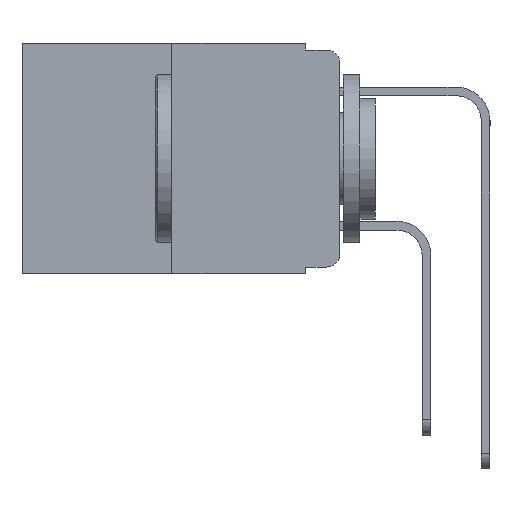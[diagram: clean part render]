
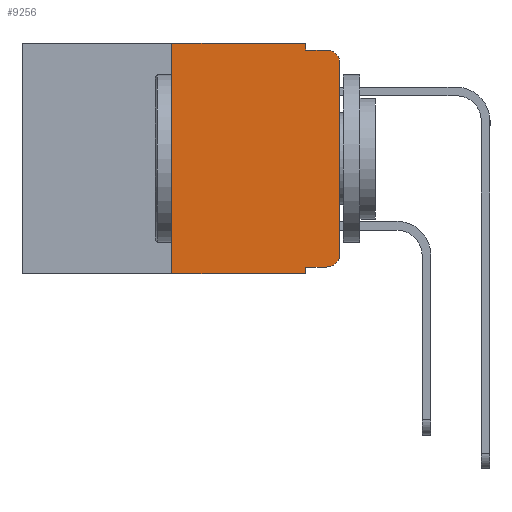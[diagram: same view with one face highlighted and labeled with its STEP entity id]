
A CAD part, left-side view. The second image highlights one B-rep face of the part: STEP entity #9256.
In plain terms, the highlighted planar face has unit normal (-1, 0, 0).
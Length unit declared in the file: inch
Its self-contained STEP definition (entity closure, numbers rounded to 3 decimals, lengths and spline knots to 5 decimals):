
#38 = LINE ( 'NONE', #16560, #7123 ) ;
#275 = CARTESIAN_POINT ( 'NONE',  ( 0., 0., 0. ) ) ;
#392 = LINE ( 'NONE', #10091, #4179 ) ;
#503 = EDGE_CURVE ( 'NONE', #14388, #8010, #17808, .T. ) ;
#567 = DIRECTION ( 'NONE',  ( 0., 0., -1. ) ) ;
#892 = EDGE_CURVE ( 'NONE', #16845, #3179, #9210, .T. ) ;
#1469 = CARTESIAN_POINT ( 'NONE',  ( 0., 0.473, 0. ) ) ;
#1489 = EDGE_CURVE ( 'NONE', #12962, #1530, #3821, .T. ) ;
#1524 = EDGE_CURVE ( 'NONE', #1530, #16485, #10267, .T. ) ;
#1530 = VERTEX_POINT ( 'NONE', #8694 ) ;
#1806 = DIRECTION ( 'NONE',  ( 0., 0., 1. ) ) ;
#2281 = ORIENTED_EDGE ( 'NONE', *, *, #11117, .T. ) ;
#2310 = VECTOR ( 'NONE', #11125, 39.37008 ) ;
#2335 = DIRECTION ( 'NONE',  ( 0., -1., 0. ) ) ;
#2382 = VERTEX_POINT ( 'NONE', #11726 ) ;
#2579 = EDGE_CURVE ( 'NONE', #4238, #16485, #3986, .T. ) ;
#2653 = DIRECTION ( 'NONE',  ( 0., 0., -1. ) ) ;
#3179 = VERTEX_POINT ( 'NONE', #8349 ) ;
#3745 = PLANE ( 'NONE',  #5446 ) ;
#3762 = ORIENTED_EDGE ( 'NONE', *, *, #15750, .T. ) ;
#3821 = LINE ( 'NONE', #16135, #18017 ) ;
#3986 = CIRCLE ( 'NONE', #4116, 0.02 ) ;
#4116 = AXIS2_PLACEMENT_3D ( 'NONE', #7783, #17404, #9135 ) ;
#4147 = EDGE_LOOP ( 'NONE', ( #3762, #6374, #8933, #12017, #14622, #15057, #10243, #17996, #2281, #17378 ) ) ;
#4179 = VECTOR ( 'NONE', #15707, 39.37008 ) ;
#4238 = VERTEX_POINT ( 'NONE', #8199 ) ;
#4444 = VECTOR ( 'NONE', #17534, 39.37008 ) ;
#5118 = CARTESIAN_POINT ( 'NONE',  ( 0., 0.473, 0. ) ) ;
#5242 = AXIS2_PLACEMENT_3D ( 'NONE', #10008, #9946, #567 ) ;
#5446 = AXIS2_PLACEMENT_3D ( 'NONE', #5118, #6543, #16204 ) ;
#5503 = EDGE_CURVE ( 'NONE', #14388, #15433, #15081, .T. ) ;
#6374 = ORIENTED_EDGE ( 'NONE', *, *, #2579, .T. ) ;
#6543 = DIRECTION ( 'NONE',  ( 1., 0., 0. ) ) ;
#6644 = CARTESIAN_POINT ( 'NONE',  ( 0., 0.051, -0.01 ) ) ;
#6838 = CARTESIAN_POINT ( 'NONE',  ( 0., 0.25, 0. ) ) ;
#7123 = VECTOR ( 'NONE', #17906, 39.37008 ) ;
#7774 = CARTESIAN_POINT ( 'NONE',  ( 0., 0.02, -0.333 ) ) ;
#7783 = CARTESIAN_POINT ( 'NONE',  ( 0., 0.02, -0.03 ) ) ;
#7862 = VECTOR ( 'NONE', #1806, 39.37008 ) ;
#7915 = CARTESIAN_POINT ( 'NONE',  ( 0., 0.473, -0.343 ) ) ;
#8010 = VERTEX_POINT ( 'NONE', #16064 ) ;
#8019 = CARTESIAN_POINT ( 'NONE',  ( 0., 0.051, -0.343 ) ) ;
#8199 = CARTESIAN_POINT ( 'NONE',  ( 0., 0., -0.03 ) ) ;
#8349 = CARTESIAN_POINT ( 'NONE',  ( 0., 0., -0.313 ) ) ;
#8694 = CARTESIAN_POINT ( 'NONE',  ( 0., 0.051, -0.01 ) ) ;
#8933 = ORIENTED_EDGE ( 'NONE', *, *, #1524, .F. ) ;
#9135 = DIRECTION ( 'NONE',  ( 0., 0., -1. ) ) ;
#9210 = CIRCLE ( 'NONE', #5242, 0.02 ) ;
#9256 = ADVANCED_FACE ( 'NONE', ( #12350 ), #3745, .F. ) ;
#9423 = DIRECTION ( 'NONE',  ( 0., 0., 1. ) ) ;
#9616 = LINE ( 'NONE', #1469, #2310 ) ;
#9946 = DIRECTION ( 'NONE',  ( -1., 0., 0. ) ) ;
#10008 = CARTESIAN_POINT ( 'NONE',  ( 0., 0.02, -0.313 ) ) ;
#10022 = CARTESIAN_POINT ( 'NONE',  ( 0., 0.25, -0.343 ) ) ;
#10091 = CARTESIAN_POINT ( 'NONE',  ( 0., 0.051, 0. ) ) ;
#10243 = ORIENTED_EDGE ( 'NONE', *, *, #5503, .T. ) ;
#10267 = LINE ( 'NONE', #6644, #17173 ) ;
#10496 = VECTOR ( 'NONE', #9423, 39.37008 ) ;
#11117 = EDGE_CURVE ( 'NONE', #2382, #16845, #38, .T. ) ;
#11125 = DIRECTION ( 'NONE',  ( 0., -1., 0. ) ) ;
#11548 = LINE ( 'NONE', #275, #7862 ) ;
#11612 = CARTESIAN_POINT ( 'NONE',  ( 0., 0.051, 0. ) ) ;
#11726 = CARTESIAN_POINT ( 'NONE',  ( 0., 0.051, -0.333 ) ) ;
#12017 = ORIENTED_EDGE ( 'NONE', *, *, #1489, .F. ) ;
#12350 = FACE_OUTER_BOUND ( 'NONE', #4147, .T. ) ;
#12962 = VERTEX_POINT ( 'NONE', #11612 ) ;
#13095 = EDGE_CURVE ( 'NONE', #8010, #12962, #9616, .T. ) ;
#13962 = CARTESIAN_POINT ( 'NONE',  ( 0., 0.02, -0.01 ) ) ;
#14388 = VERTEX_POINT ( 'NONE', #10022 ) ;
#14622 = ORIENTED_EDGE ( 'NONE', *, *, #13095, .F. ) ;
#15057 = ORIENTED_EDGE ( 'NONE', *, *, #503, .F. ) ;
#15081 = LINE ( 'NONE', #7915, #4444 ) ;
#15433 = VERTEX_POINT ( 'NONE', #8019 ) ;
#15707 = DIRECTION ( 'NONE',  ( 0., 0., -1. ) ) ;
#15750 = EDGE_CURVE ( 'NONE', #3179, #4238, #11548, .T. ) ;
#15782 = EDGE_CURVE ( 'NONE', #2382, #15433, #392, .T. ) ;
#16064 = CARTESIAN_POINT ( 'NONE',  ( 0., 0.25, 0. ) ) ;
#16135 = CARTESIAN_POINT ( 'NONE',  ( 0., 0.051, 0. ) ) ;
#16204 = DIRECTION ( 'NONE',  ( 0., 0., -1. ) ) ;
#16485 = VERTEX_POINT ( 'NONE', #13962 ) ;
#16560 = CARTESIAN_POINT ( 'NONE',  ( 0., 0.051, -0.333 ) ) ;
#16845 = VERTEX_POINT ( 'NONE', #7774 ) ;
#17173 = VECTOR ( 'NONE', #2335, 39.37008 ) ;
#17378 = ORIENTED_EDGE ( 'NONE', *, *, #892, .T. ) ;
#17404 = DIRECTION ( 'NONE',  ( -1., 0., 0. ) ) ;
#17534 = DIRECTION ( 'NONE',  ( 0., -1., 0. ) ) ;
#17808 = LINE ( 'NONE', #6838, #10496 ) ;
#17906 = DIRECTION ( 'NONE',  ( 0., -1., 0. ) ) ;
#17996 = ORIENTED_EDGE ( 'NONE', *, *, #15782, .F. ) ;
#18017 = VECTOR ( 'NONE', #2653, 39.37008 ) ;
